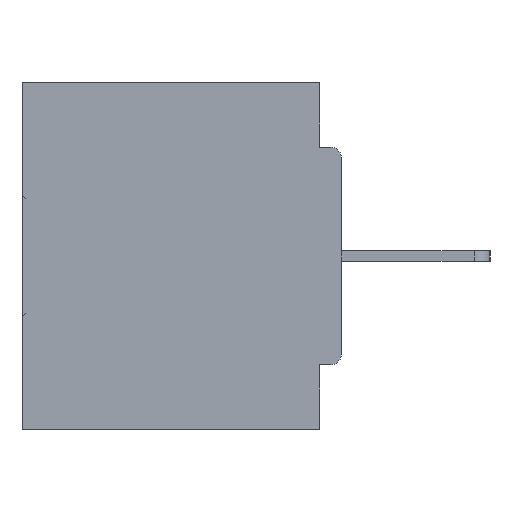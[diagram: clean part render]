
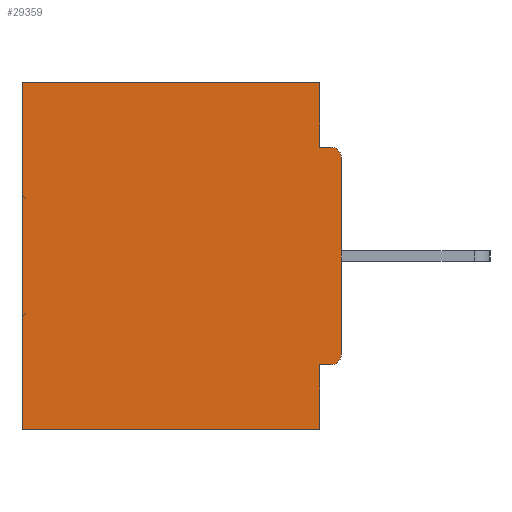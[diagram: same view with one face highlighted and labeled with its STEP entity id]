
A CAD part, left-side view. The second image highlights one B-rep face of the part: STEP entity #29359.
In plain terms, the highlighted planar face has unit normal (-1, 0, 0).
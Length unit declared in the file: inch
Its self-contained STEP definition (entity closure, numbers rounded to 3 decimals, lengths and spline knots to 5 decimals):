
#1253 = DIRECTION ( 'NONE',  ( 0., 0., -1. ) ) ;
#1474 = VERTEX_POINT ( 'NONE', #36461 ) ;
#1548 = DIRECTION ( 'NONE',  ( 1., 0., 0. ) ) ;
#2311 = ORIENTED_EDGE ( 'NONE', *, *, #34256, .T. ) ;
#2700 = DIRECTION ( 'NONE',  ( 0., 1., 0. ) ) ;
#3517 = EDGE_CURVE ( 'NONE', #14748, #19583, #24430, .T. ) ;
#5539 = VERTEX_POINT ( 'NONE', #29854 ) ;
#6757 = CARTESIAN_POINT ( 'NONE',  ( 0.298, 0., 0. ) ) ;
#7219 = DIRECTION ( 'NONE',  ( -1., 0., 0. ) ) ;
#8159 = LINE ( 'NONE', #20151, #26413 ) ;
#8656 = CARTESIAN_POINT ( 'NONE',  ( 0.298, 0., -0.0935 ) ) ;
#8892 = LINE ( 'NONE', #11808, #32436 ) ;
#9345 = EDGE_LOOP ( 'NONE', ( #38588, #35178, #25233, #33071, #2311, #13257, #27139, #18843, #14938, #32759 ) ) ;
#9764 = VECTOR ( 'NONE', #1253, 39.37008 ) ;
#10386 = CARTESIAN_POINT ( 'NONE',  ( 0.298, 0., 0. ) ) ;
#10666 = CARTESIAN_POINT ( 'NONE',  ( 0.298, 0., 0. ) ) ;
#11534 = LINE ( 'NONE', #26704, #37249 ) ;
#11686 = CARTESIAN_POINT ( 'NONE',  ( 0.298, 0.031, 0. ) ) ;
#11808 = CARTESIAN_POINT ( 'NONE',  ( 0.298, 0.46, 0. ) ) ;
#12036 = CARTESIAN_POINT ( 'NONE',  ( 0.298, 0.46, -0.5 ) ) ;
#12180 = VECTOR ( 'NONE', #26754, 39.37008 ) ;
#12220 = CARTESIAN_POINT ( 'NONE',  ( 0.298, 0., -0.3915 ) ) ;
#12258 = CARTESIAN_POINT ( 'NONE',  ( 0.298, 0.015, -0.0935 ) ) ;
#12332 = CARTESIAN_POINT ( 'NONE',  ( 0.298, 0., -0.1085 ) ) ;
#12954 = LINE ( 'NONE', #28343, #14026 ) ;
#13257 = ORIENTED_EDGE ( 'NONE', *, *, #35103, .F. ) ;
#13713 = DIRECTION ( 'NONE',  ( 0., 0., -1. ) ) ;
#14026 = VECTOR ( 'NONE', #13713, 39.37008 ) ;
#14748 = VERTEX_POINT ( 'NONE', #12332 ) ;
#14749 = DIRECTION ( 'NONE',  ( 0., 0., -1. ) ) ;
#14938 = ORIENTED_EDGE ( 'NONE', *, *, #19445, .T. ) ;
#16195 = EDGE_CURVE ( 'NONE', #35283, #16766, #11534, .T. ) ;
#16766 = VERTEX_POINT ( 'NONE', #33874 ) ;
#17027 = AXIS2_PLACEMENT_3D ( 'NONE', #22940, #7219, #19195 ) ;
#17260 = VERTEX_POINT ( 'NONE', #22409 ) ;
#17417 = CARTESIAN_POINT ( 'NONE',  ( 0.298, 0., -0.5 ) ) ;
#17476 = LINE ( 'NONE', #8656, #12180 ) ;
#18598 = DIRECTION ( 'NONE',  ( -1., 0., 0. ) ) ;
#18843 = ORIENTED_EDGE ( 'NONE', *, *, #16195, .F. ) ;
#19195 = DIRECTION ( 'NONE',  ( 0., 0., -1. ) ) ;
#19445 = EDGE_CURVE ( 'NONE', #35283, #21280, #38400, .T. ) ;
#19583 = VERTEX_POINT ( 'NONE', #12258 ) ;
#19608 = DIRECTION ( 'NONE',  ( 0., 0., -1. ) ) ;
#20151 = CARTESIAN_POINT ( 'NONE',  ( 0.298, 0.031, -0.5 ) ) ;
#21280 = VERTEX_POINT ( 'NONE', #12220 ) ;
#21808 = EDGE_CURVE ( 'NONE', #25781, #5539, #12954, .T. ) ;
#22373 = VERTEX_POINT ( 'NONE', #12036 ) ;
#22409 = CARTESIAN_POINT ( 'NONE',  ( 0.298, 0.031, -0.5 ) ) ;
#22474 = EDGE_CURVE ( 'NONE', #25781, #1474, #30742, .T. ) ;
#22694 = EDGE_CURVE ( 'NONE', #14748, #21280, #28197, .T. ) ;
#22734 = DIRECTION ( 'NONE',  ( 0., 0., -1. ) ) ;
#22940 = CARTESIAN_POINT ( 'NONE',  ( 0.298, 0.015, -0.3915 ) ) ;
#23671 = EDGE_CURVE ( 'NONE', #5539, #19583, #17476, .T. ) ;
#24176 = VECTOR ( 'NONE', #28000, 39.37008 ) ;
#24430 = CIRCLE ( 'NONE', #34465, 0.015 ) ;
#25233 = ORIENTED_EDGE ( 'NONE', *, *, #21808, .F. ) ;
#25781 = VERTEX_POINT ( 'NONE', #11686 ) ;
#26413 = VECTOR ( 'NONE', #22734, 39.37008 ) ;
#26704 = CARTESIAN_POINT ( 'NONE',  ( 0.298, 0., -0.4065 ) ) ;
#26754 = DIRECTION ( 'NONE',  ( 0., -1., 0. ) ) ;
#27139 = ORIENTED_EDGE ( 'NONE', *, *, #29958, .F. ) ;
#28000 = DIRECTION ( 'NONE',  ( 0., 1., 0. ) ) ;
#28197 = LINE ( 'NONE', #10666, #9764 ) ;
#28259 = CARTESIAN_POINT ( 'NONE',  ( 0.298, 0.015, -0.4065 ) ) ;
#28343 = CARTESIAN_POINT ( 'NONE',  ( 0.298, 0.031, -0.5 ) ) ;
#28694 = FACE_OUTER_BOUND ( 'NONE', #9345, .T. ) ;
#29359 = ADVANCED_FACE ( 'NONE', ( #28694 ), #37320, .F. ) ;
#29461 = DIRECTION ( 'NONE',  ( 0., 1., 0. ) ) ;
#29854 = CARTESIAN_POINT ( 'NONE',  ( 0.298, 0.031, -0.0935 ) ) ;
#29958 = EDGE_CURVE ( 'NONE', #16766, #17260, #8159, .T. ) ;
#30530 = VECTOR ( 'NONE', #29461, 39.37008 ) ;
#30742 = LINE ( 'NONE', #6757, #24176 ) ;
#30799 = DIRECTION ( 'NONE',  ( 0., 0., -1. ) ) ;
#32390 = LINE ( 'NONE', #17417, #30530 ) ;
#32436 = VECTOR ( 'NONE', #14749, 39.37008 ) ;
#32759 = ORIENTED_EDGE ( 'NONE', *, *, #22694, .F. ) ;
#33071 = ORIENTED_EDGE ( 'NONE', *, *, #22474, .T. ) ;
#33178 = AXIS2_PLACEMENT_3D ( 'NONE', #10386, #1548, #19608 ) ;
#33874 = CARTESIAN_POINT ( 'NONE',  ( 0.298, 0.031, -0.4065 ) ) ;
#34256 = EDGE_CURVE ( 'NONE', #1474, #22373, #8892, .T. ) ;
#34465 = AXIS2_PLACEMENT_3D ( 'NONE', #36895, #18598, #30799 ) ;
#35103 = EDGE_CURVE ( 'NONE', #17260, #22373, #32390, .T. ) ;
#35178 = ORIENTED_EDGE ( 'NONE', *, *, #23671, .F. ) ;
#35283 = VERTEX_POINT ( 'NONE', #28259 ) ;
#36461 = CARTESIAN_POINT ( 'NONE',  ( 0.298, 0.46, 0. ) ) ;
#36895 = CARTESIAN_POINT ( 'NONE',  ( 0.298, 0.015, -0.1085 ) ) ;
#37249 = VECTOR ( 'NONE', #2700, 39.37008 ) ;
#37320 = PLANE ( 'NONE',  #33178 ) ;
#38400 = CIRCLE ( 'NONE', #17027, 0.015 ) ;
#38588 = ORIENTED_EDGE ( 'NONE', *, *, #3517, .T. ) ;
